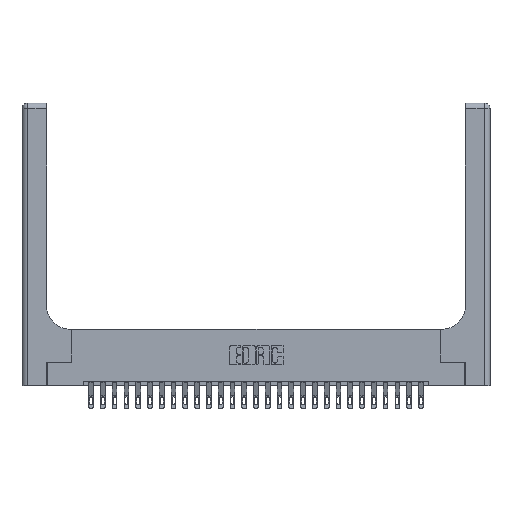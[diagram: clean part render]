
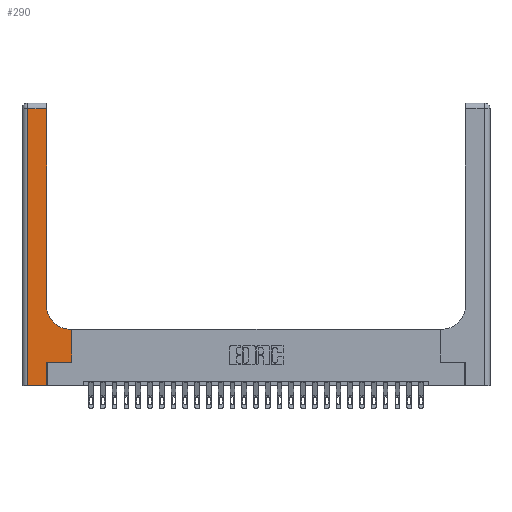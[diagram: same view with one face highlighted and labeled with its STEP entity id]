
A CAD part, top view. The second image highlights one B-rep face of the part: STEP entity #290.
In plain terms, the highlighted planar face has unit normal (0, 0, 1).
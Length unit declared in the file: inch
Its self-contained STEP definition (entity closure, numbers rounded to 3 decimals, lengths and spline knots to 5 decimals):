
#290 = ADVANCED_FACE ( 'NONE', ( #17091 ), #2210, .F. ) ;
#883 = ORIENTED_EDGE ( 'NONE', *, *, #6166, .T. ) ;
#1646 = CARTESIAN_POINT ( 'NONE',  ( 0.26, 0.85, 0.37 ) ) ;
#1926 = VERTEX_POINT ( 'NONE', #19445 ) ;
#2210 = PLANE ( 'NONE',  #10250 ) ;
#2476 = CARTESIAN_POINT ( 'NONE',  ( 0.51, 0.6, 0.37 ) ) ;
#2539 = EDGE_CURVE ( 'NONE', #4698, #4359, #18542, .T. ) ;
#2564 = CARTESIAN_POINT ( 'NONE',  ( 0., 3., 0.37 ) ) ;
#2927 = LINE ( 'NONE', #22321, #14904 ) ;
#2938 = ORIENTED_EDGE ( 'NONE', *, *, #2539, .T. ) ;
#3243 = CARTESIAN_POINT ( 'NONE',  ( 0.528, 0.25, 0.37 ) ) ;
#3579 = LINE ( 'NONE', #9577, #24446 ) ;
#4359 = VERTEX_POINT ( 'NONE', #15274 ) ;
#4698 = VERTEX_POINT ( 'NONE', #4797 ) ;
#4797 = CARTESIAN_POINT ( 'NONE',  ( 0.26, 2.94, 0.37 ) ) ;
#5461 = VECTOR ( 'NONE', #10420, 39.37008 ) ;
#5492 = LINE ( 'NONE', #20069, #14314 ) ;
#6166 = EDGE_CURVE ( 'NONE', #24123, #4698, #2927, .T. ) ;
#6286 = EDGE_CURVE ( 'NONE', #10254, #15305, #26006, .T. ) ;
#6480 = DIRECTION ( 'NONE',  ( -1., 0., 0. ) ) ;
#6882 = CIRCLE ( 'NONE', #24574, 0.25 ) ;
#6928 = ORIENTED_EDGE ( 'NONE', *, *, #12810, .T. ) ;
#7647 = EDGE_CURVE ( 'NONE', #23761, #24123, #6882, .T. ) ;
#8003 = DIRECTION ( 'NONE',  ( 1., 0., 0. ) ) ;
#8649 = EDGE_LOOP ( 'NONE', ( #883, #2938, #15628, #6928, #24053, #18134, #24761, #22248, #8693 ) ) ;
#8693 = ORIENTED_EDGE ( 'NONE', *, *, #7647, .T. ) ;
#9283 = VERTEX_POINT ( 'NONE', #23699 ) ;
#9356 = DIRECTION ( 'NONE',  ( 0., 1., 0. ) ) ;
#9577 = CARTESIAN_POINT ( 'NONE',  ( 0.26, 0.6, 0.37 ) ) ;
#10250 = AXIS2_PLACEMENT_3D ( 'NONE', #2564, #18450, #24686 ) ;
#10254 = VERTEX_POINT ( 'NONE', #20622 ) ;
#10420 = DIRECTION ( 'NONE',  ( 0., 1., 0. ) ) ;
#10889 = EDGE_CURVE ( 'NONE', #15305, #25007, #5492, .T. ) ;
#11379 = DIRECTION ( 'NONE',  ( 0., -1., 0. ) ) ;
#12641 = VECTOR ( 'NONE', #11379, 39.37008 ) ;
#12810 = EDGE_CURVE ( 'NONE', #1926, #10254, #13266, .T. ) ;
#12853 = EDGE_CURVE ( 'NONE', #4359, #1926, #13911, .T. ) ;
#12961 = DIRECTION ( 'NONE',  ( 0., 0., -1. ) ) ;
#13135 = DIRECTION ( 'NONE',  ( 1., 0., 0. ) ) ;
#13266 = LINE ( 'NONE', #19649, #14842 ) ;
#13911 = LINE ( 'NONE', #25688, #12641 ) ;
#14314 = VECTOR ( 'NONE', #8003, 39.37008 ) ;
#14357 = CARTESIAN_POINT ( 'NONE',  ( 0.265, 0., 0.37 ) ) ;
#14842 = VECTOR ( 'NONE', #19565, 39.37008 ) ;
#14904 = VECTOR ( 'NONE', #18248, 39.37008 ) ;
#15274 = CARTESIAN_POINT ( 'NONE',  ( 0.06, 2.94, 0.37 ) ) ;
#15305 = VERTEX_POINT ( 'NONE', #22760 ) ;
#15628 = ORIENTED_EDGE ( 'NONE', *, *, #12853, .T. ) ;
#16269 = EDGE_CURVE ( 'NONE', #9283, #23761, #3579, .T. ) ;
#16633 = VECTOR ( 'NONE', #6480, 39.37008 ) ;
#17091 = FACE_OUTER_BOUND ( 'NONE', #8649, .T. ) ;
#17405 = DIRECTION ( 'NONE',  ( -1., 0., 0. ) ) ;
#18134 = ORIENTED_EDGE ( 'NONE', *, *, #10889, .T. ) ;
#18248 = DIRECTION ( 'NONE',  ( 0., 1., 0. ) ) ;
#18373 = CARTESIAN_POINT ( 'NONE',  ( 0.528, 0.25, 0.37 ) ) ;
#18450 = DIRECTION ( 'NONE',  ( 0., 0., -1. ) ) ;
#18542 = LINE ( 'NONE', #24332, #16633 ) ;
#19139 = CARTESIAN_POINT ( 'NONE',  ( 0.51, 0.85, 0.37 ) ) ;
#19189 = LINE ( 'NONE', #3243, #24309 ) ;
#19445 = CARTESIAN_POINT ( 'NONE',  ( 0.06, 0., 0.37 ) ) ;
#19565 = DIRECTION ( 'NONE',  ( 1., 0., 0. ) ) ;
#19649 = CARTESIAN_POINT ( 'NONE',  ( 0., 0., 0.37 ) ) ;
#20069 = CARTESIAN_POINT ( 'NONE',  ( 0.265, 0.25, 0.37 ) ) ;
#20622 = CARTESIAN_POINT ( 'NONE',  ( 0.265, 0., 0.37 ) ) ;
#20827 = EDGE_CURVE ( 'NONE', #25007, #9283, #19189, .T. ) ;
#22248 = ORIENTED_EDGE ( 'NONE', *, *, #16269, .T. ) ;
#22321 = CARTESIAN_POINT ( 'NONE',  ( 0.26, 3., 0.37 ) ) ;
#22760 = CARTESIAN_POINT ( 'NONE',  ( 0.265, 0.25, 0.37 ) ) ;
#23699 = CARTESIAN_POINT ( 'NONE',  ( 0.528, 0.6, 0.37 ) ) ;
#23761 = VERTEX_POINT ( 'NONE', #2476 ) ;
#24053 = ORIENTED_EDGE ( 'NONE', *, *, #6286, .T. ) ;
#24123 = VERTEX_POINT ( 'NONE', #1646 ) ;
#24309 = VECTOR ( 'NONE', #9356, 39.37008 ) ;
#24332 = CARTESIAN_POINT ( 'NONE',  ( 0., 2.94, 0.37 ) ) ;
#24446 = VECTOR ( 'NONE', #17405, 39.37008 ) ;
#24574 = AXIS2_PLACEMENT_3D ( 'NONE', #19139, #12961, #13135 ) ;
#24686 = DIRECTION ( 'NONE',  ( -1., 0., 0. ) ) ;
#24761 = ORIENTED_EDGE ( 'NONE', *, *, #20827, .T. ) ;
#25007 = VERTEX_POINT ( 'NONE', #18373 ) ;
#25688 = CARTESIAN_POINT ( 'NONE',  ( 0.06, 3., 0.37 ) ) ;
#26006 = LINE ( 'NONE', #14357, #5461 ) ;
